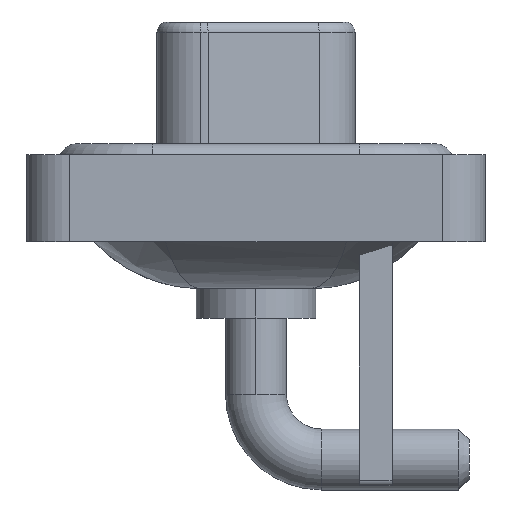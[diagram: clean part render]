
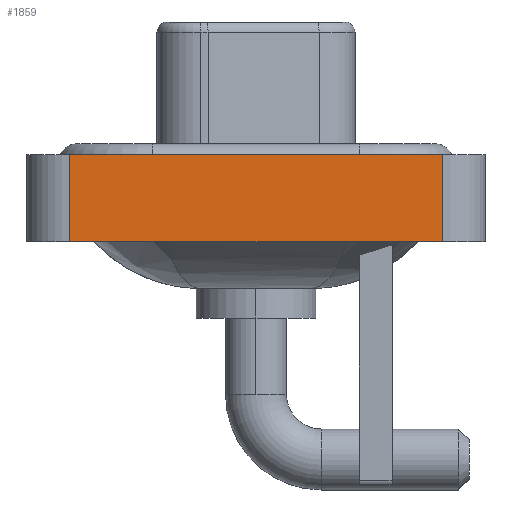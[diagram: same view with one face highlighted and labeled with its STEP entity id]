
A CAD part, left-side view. The second image highlights one B-rep face of the part: STEP entity #1859.
In plain terms, the highlighted planar face has unit normal (-1, 0, 0).
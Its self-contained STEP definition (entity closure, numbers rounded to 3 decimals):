
#443 = EDGE_LOOP ( 'NONE', ( #14103, #5460, #10654, #12917 ) ) ;
#564 = FACE_OUTER_BOUND ( 'NONE', #443, .T. ) ;
#642 = DIRECTION ( 'NONE',  ( 0., 0., 1. ) ) ;
#713 = VECTOR ( 'NONE', #9867, 1000. ) ;
#1172 = EDGE_CURVE ( 'NONE', #9614, #9158, #1378, .T. ) ;
#1309 = CARTESIAN_POINT ( 'NONE',  ( -7.25, -8.55, 0.4 ) ) ;
#1378 = LINE ( 'NONE', #2419, #713 ) ;
#1859 = ADVANCED_FACE ( 'NONE', ( #564 ), #11675, .T. ) ;
#2183 = EDGE_CURVE ( 'NONE', #13643, #9158, #7725, .T. ) ;
#2419 = CARTESIAN_POINT ( 'NONE',  ( -7.25, -8.55, 0.4 ) ) ;
#4884 = LINE ( 'NONE', #14504, #9816 ) ;
#5073 = AXIS2_PLACEMENT_3D ( 'NONE', #15295, #8004, #642 ) ;
#5460 = ORIENTED_EDGE ( 'NONE', *, *, #1172, .F. ) ;
#5486 = CARTESIAN_POINT ( 'NONE',  ( -7.25, -8.55, -3.6 ) ) ;
#5546 = CARTESIAN_POINT ( 'NONE',  ( -7.25, 8.55, 0.4 ) ) ;
#7433 = LINE ( 'NONE', #13445, #8595 ) ;
#7725 = LINE ( 'NONE', #5486, #12982 ) ;
#8004 = DIRECTION ( 'NONE',  ( -1., 0., 0. ) ) ;
#8595 = VECTOR ( 'NONE', #12240, 1000. ) ;
#9158 = VERTEX_POINT ( 'NONE', #1309 ) ;
#9261 = CARTESIAN_POINT ( 'NONE',  ( -7.25, -8.55, -3.6 ) ) ;
#9614 = VERTEX_POINT ( 'NONE', #5546 ) ;
#9777 = EDGE_CURVE ( 'NONE', #14600, #9614, #4884, .T. ) ;
#9816 = VECTOR ( 'NONE', #12016, 1000. ) ;
#9867 = DIRECTION ( 'NONE',  ( 0., -1., 0. ) ) ;
#10654 = ORIENTED_EDGE ( 'NONE', *, *, #9777, .F. ) ;
#11675 = PLANE ( 'NONE',  #5073 ) ;
#11696 = EDGE_CURVE ( 'NONE', #14600, #13643, #7433, .T. ) ;
#12016 = DIRECTION ( 'NONE',  ( 0., 0., 1. ) ) ;
#12240 = DIRECTION ( 'NONE',  ( 0., -1., 0. ) ) ;
#12857 = DIRECTION ( 'NONE',  ( 0., 0., 1. ) ) ;
#12891 = CARTESIAN_POINT ( 'NONE',  ( -7.25, 8.55, -3.6 ) ) ;
#12917 = ORIENTED_EDGE ( 'NONE', *, *, #11696, .T. ) ;
#12982 = VECTOR ( 'NONE', #12857, 1000. ) ;
#13445 = CARTESIAN_POINT ( 'NONE',  ( -7.25, -8.55, -3.6 ) ) ;
#13643 = VERTEX_POINT ( 'NONE', #9261 ) ;
#14103 = ORIENTED_EDGE ( 'NONE', *, *, #2183, .T. ) ;
#14504 = CARTESIAN_POINT ( 'NONE',  ( -7.25, 8.55, -3.6 ) ) ;
#14600 = VERTEX_POINT ( 'NONE', #12891 ) ;
#15295 = CARTESIAN_POINT ( 'NONE',  ( -7.25, -8.55, -3.6 ) ) ;
